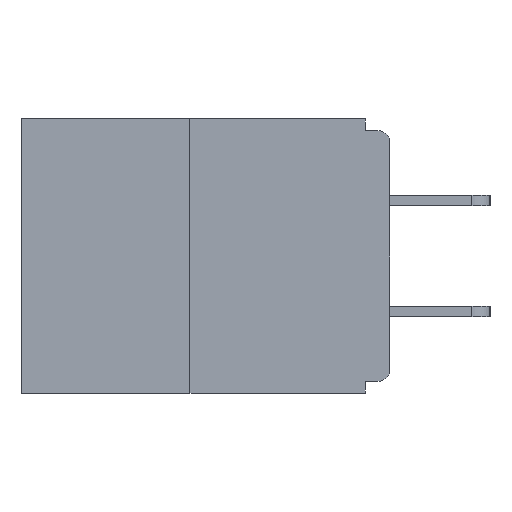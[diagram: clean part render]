
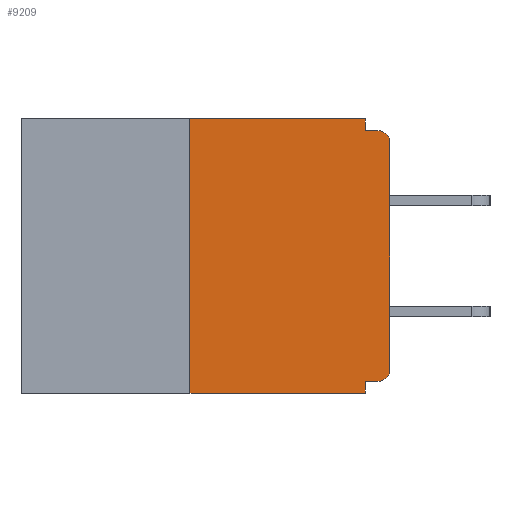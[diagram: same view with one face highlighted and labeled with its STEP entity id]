
A CAD part, left-side view. The second image highlights one B-rep face of the part: STEP entity #9209.
In plain terms, the highlighted planar face has unit normal (-1, 0, 0).
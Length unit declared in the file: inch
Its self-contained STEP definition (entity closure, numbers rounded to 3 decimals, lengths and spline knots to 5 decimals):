
#196 = ORIENTED_EDGE ( 'NONE', *, *, #4548, .F. ) ;
#287 = VERTEX_POINT ( 'NONE', #6692 ) ;
#601 = EDGE_LOOP ( 'NONE', ( #196, #15704, #5278, #18402, #3213, #18035, #10997, #18470, #8195, #2989 ) ) ;
#621 = VECTOR ( 'NONE', #7192, 39.37008 ) ;
#639 = CARTESIAN_POINT ( 'NONE',  ( 0., 0.25, -0.343 ) ) ;
#694 = DIRECTION ( 'NONE',  ( 0., 0., -1. ) ) ;
#1670 = AXIS2_PLACEMENT_3D ( 'NONE', #11978, #7579, #1980 ) ;
#1760 = CARTESIAN_POINT ( 'NONE',  ( 0., 0.031, -0.328 ) ) ;
#1980 = DIRECTION ( 'NONE',  ( 0., 0., -1. ) ) ;
#2027 = DIRECTION ( 'NONE',  ( -1., 0., 0. ) ) ;
#2065 = DIRECTION ( 'NONE',  ( 0., -1., 0. ) ) ;
#2081 = CARTESIAN_POINT ( 'NONE',  ( 0., 0.25, 0. ) ) ;
#2813 = EDGE_CURVE ( 'NONE', #13211, #10488, #6428, .T. ) ;
#2989 = ORIENTED_EDGE ( 'NONE', *, *, #12397, .F. ) ;
#3213 = ORIENTED_EDGE ( 'NONE', *, *, #11175, .F. ) ;
#3596 = VERTEX_POINT ( 'NONE', #1760 ) ;
#3810 = DIRECTION ( 'NONE',  ( 0., -1., 0. ) ) ;
#4052 = CARTESIAN_POINT ( 'NONE',  ( 0., 0.031, -0.015 ) ) ;
#4392 = AXIS2_PLACEMENT_3D ( 'NONE', #6379, #12209, #694 ) ;
#4422 = CARTESIAN_POINT ( 'NONE',  ( 0., 0., 0. ) ) ;
#4548 = EDGE_CURVE ( 'NONE', #10488, #6055, #17634, .T. ) ;
#4983 = CARTESIAN_POINT ( 'NONE',  ( 0., 0.25, 0. ) ) ;
#5124 = LINE ( 'NONE', #18150, #18883 ) ;
#5278 = ORIENTED_EDGE ( 'NONE', *, *, #18438, .T. ) ;
#5375 = VERTEX_POINT ( 'NONE', #12814 ) ;
#6038 = CARTESIAN_POINT ( 'NONE',  ( 0., 0.46, 0. ) ) ;
#6055 = VERTEX_POINT ( 'NONE', #12485 ) ;
#6173 = VERTEX_POINT ( 'NONE', #12582 ) ;
#6328 = EDGE_CURVE ( 'NONE', #12270, #16316, #14680, .T. ) ;
#6379 = CARTESIAN_POINT ( 'NONE',  ( 0., 0.015, -0.313 ) ) ;
#6428 = LINE ( 'NONE', #2081, #12024 ) ;
#6470 = CARTESIAN_POINT ( 'NONE',  ( 0., 0.031, -0.343 ) ) ;
#6521 = DIRECTION ( 'NONE',  ( 0., 0., 1. ) ) ;
#6692 = CARTESIAN_POINT ( 'NONE',  ( 0., 0.015, -0.328 ) ) ;
#7192 = DIRECTION ( 'NONE',  ( 0., 0., 1. ) ) ;
#7409 = VECTOR ( 'NONE', #7481, 39.37008 ) ;
#7481 = DIRECTION ( 'NONE',  ( 0., -1., 0. ) ) ;
#7482 = FACE_OUTER_BOUND ( 'NONE', #601, .T. ) ;
#7579 = DIRECTION ( 'NONE',  ( 1., 0., 0. ) ) ;
#7591 = DIRECTION ( 'NONE',  ( 0., 0., -1. ) ) ;
#7873 = EDGE_CURVE ( 'NONE', #5375, #6173, #14375, .T. ) ;
#7908 = DIRECTION ( 'NONE',  ( 0., 0., -1. ) ) ;
#8195 = ORIENTED_EDGE ( 'NONE', *, *, #6328, .F. ) ;
#8666 = CARTESIAN_POINT ( 'NONE',  ( 0., 0.031, -0.343 ) ) ;
#9209 = ADVANCED_FACE ( 'NONE', ( #7482 ), #12161, .F. ) ;
#9436 = CARTESIAN_POINT ( 'NONE',  ( 0., 0., -0.328 ) ) ;
#9620 = LINE ( 'NONE', #16894, #18545 ) ;
#9712 = EDGE_CURVE ( 'NONE', #6173, #16316, #16913, .T. ) ;
#9899 = AXIS2_PLACEMENT_3D ( 'NONE', #16516, #2027, #7908 ) ;
#10348 = VECTOR ( 'NONE', #7591, 39.37008 ) ;
#10488 = VERTEX_POINT ( 'NONE', #4983 ) ;
#10997 = ORIENTED_EDGE ( 'NONE', *, *, #7873, .T. ) ;
#11072 = DIRECTION ( 'NONE',  ( 0., 0., -1. ) ) ;
#11175 = EDGE_CURVE ( 'NONE', #287, #3596, #15454, .T. ) ;
#11322 = CARTESIAN_POINT ( 'NONE',  ( 0., 0.015, -0.015 ) ) ;
#11978 = CARTESIAN_POINT ( 'NONE',  ( 0., 0.46, 0. ) ) ;
#12024 = VECTOR ( 'NONE', #6521, 39.37008 ) ;
#12161 = PLANE ( 'NONE',  #1670 ) ;
#12209 = DIRECTION ( 'NONE',  ( -1., 0., 0. ) ) ;
#12270 = VERTEX_POINT ( 'NONE', #4052 ) ;
#12397 = EDGE_CURVE ( 'NONE', #6055, #12270, #5124, .T. ) ;
#12485 = CARTESIAN_POINT ( 'NONE',  ( 0., 0.031, 0. ) ) ;
#12582 = CARTESIAN_POINT ( 'NONE',  ( 0., 0., -0.03 ) ) ;
#12814 = CARTESIAN_POINT ( 'NONE',  ( 0., 0., -0.313 ) ) ;
#13211 = VERTEX_POINT ( 'NONE', #639 ) ;
#14023 = DIRECTION ( 'NONE',  ( 0., 1., 0. ) ) ;
#14375 = LINE ( 'NONE', #4422, #621 ) ;
#14479 = CIRCLE ( 'NONE', #4392, 0.015 ) ;
#14680 = LINE ( 'NONE', #18006, #15016 ) ;
#14736 = EDGE_CURVE ( 'NONE', #3596, #15065, #16291, .T. ) ;
#15016 = VECTOR ( 'NONE', #2065, 39.37008 ) ;
#15051 = EDGE_CURVE ( 'NONE', #287, #5375, #14479, .T. ) ;
#15065 = VERTEX_POINT ( 'NONE', #6470 ) ;
#15454 = LINE ( 'NONE', #9436, #17587 ) ;
#15704 = ORIENTED_EDGE ( 'NONE', *, *, #2813, .F. ) ;
#16291 = LINE ( 'NONE', #8666, #10348 ) ;
#16316 = VERTEX_POINT ( 'NONE', #11322 ) ;
#16516 = CARTESIAN_POINT ( 'NONE',  ( 0., 0.015, -0.03 ) ) ;
#16894 = CARTESIAN_POINT ( 'NONE',  ( 0., 0.46, -0.343 ) ) ;
#16913 = CIRCLE ( 'NONE', #9899, 0.015 ) ;
#17587 = VECTOR ( 'NONE', #14023, 39.37008 ) ;
#17634 = LINE ( 'NONE', #6038, #7409 ) ;
#18006 = CARTESIAN_POINT ( 'NONE',  ( 0., 0., -0.015 ) ) ;
#18035 = ORIENTED_EDGE ( 'NONE', *, *, #15051, .T. ) ;
#18150 = CARTESIAN_POINT ( 'NONE',  ( 0., 0.031, 0. ) ) ;
#18402 = ORIENTED_EDGE ( 'NONE', *, *, #14736, .F. ) ;
#18438 = EDGE_CURVE ( 'NONE', #13211, #15065, #9620, .T. ) ;
#18470 = ORIENTED_EDGE ( 'NONE', *, *, #9712, .T. ) ;
#18545 = VECTOR ( 'NONE', #3810, 39.37008 ) ;
#18883 = VECTOR ( 'NONE', #11072, 39.37008 ) ;
